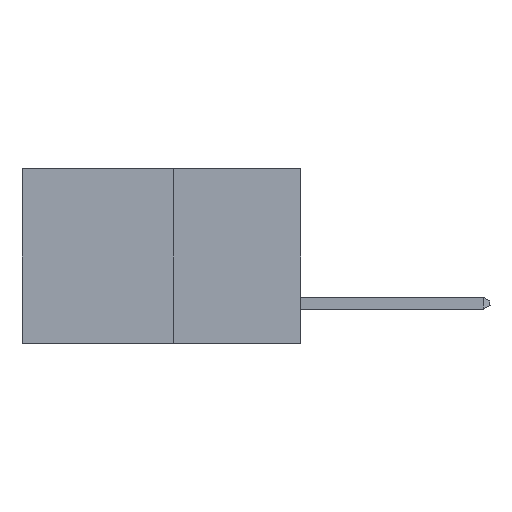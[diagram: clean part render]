
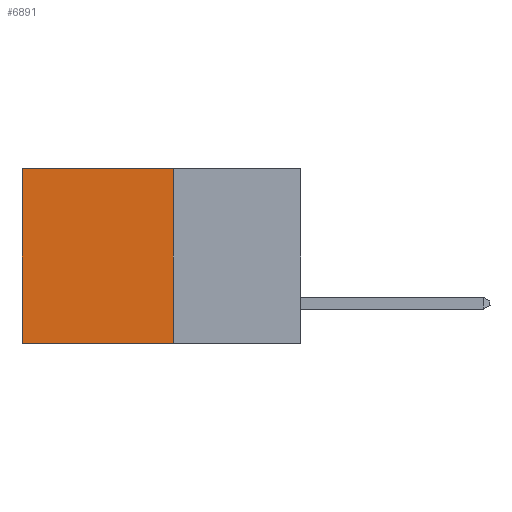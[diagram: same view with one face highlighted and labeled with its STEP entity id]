
A CAD part, left-side view. The second image highlights one B-rep face of the part: STEP entity #6891.
In plain terms, the highlighted planar face has unit normal (-1, 0, 0).
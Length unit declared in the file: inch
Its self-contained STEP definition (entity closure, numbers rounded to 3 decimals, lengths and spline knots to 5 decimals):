
#2284 = CARTESIAN_POINT ( 'NONE',  ( 0.277, 0.59, -0.37 ) ) ;
#2508 = ORIENTED_EDGE ( 'NONE', *, *, #15942, .T. ) ;
#3326 = VECTOR ( 'NONE', #10440, 39.37008 ) ;
#3743 = DIRECTION ( 'NONE',  ( 0., 0., -1. ) ) ;
#4179 = CARTESIAN_POINT ( 'NONE',  ( 0.277, 0.59, 0. ) ) ;
#4608 = FACE_OUTER_BOUND ( 'NONE', #17397, .T. ) ;
#4986 = VECTOR ( 'NONE', #6663, 39.37008 ) ;
#5102 = VERTEX_POINT ( 'NONE', #4179 ) ;
#5275 = CARTESIAN_POINT ( 'NONE',  ( 0.277, 0.27, 0. ) ) ;
#5634 = EDGE_CURVE ( 'NONE', #15242, #12633, #6999, .T. ) ;
#6340 = VECTOR ( 'NONE', #3743, 39.37008 ) ;
#6663 = DIRECTION ( 'NONE',  ( 0., 1., 0. ) ) ;
#6891 = ADVANCED_FACE ( 'NONE', ( #4608 ), #11774, .F. ) ;
#6999 = LINE ( 'NONE', #14785, #3326 ) ;
#7705 = EDGE_CURVE ( 'NONE', #15242, #5102, #15809, .T. ) ;
#9781 = DIRECTION ( 'NONE',  ( 0., 0., -1. ) ) ;
#9804 = DIRECTION ( 'NONE',  ( 1., 0., 0. ) ) ;
#9854 = CARTESIAN_POINT ( 'NONE',  ( 0.277, 0.27, -0.37 ) ) ;
#9985 = LINE ( 'NONE', #15391, #12744 ) ;
#10440 = DIRECTION ( 'NONE',  ( 0., 0., -1. ) ) ;
#10930 = EDGE_CURVE ( 'NONE', #12633, #11135, #9985, .T. ) ;
#11135 = VERTEX_POINT ( 'NONE', #14461 ) ;
#11774 = PLANE ( 'NONE',  #15640 ) ;
#12633 = VERTEX_POINT ( 'NONE', #17826 ) ;
#12744 = VECTOR ( 'NONE', #16720, 39.37008 ) ;
#13635 = LINE ( 'NONE', #2284, #6340 ) ;
#13763 = ORIENTED_EDGE ( 'NONE', *, *, #5634, .F. ) ;
#14461 = CARTESIAN_POINT ( 'NONE',  ( 0.277, 0.59, -0.37 ) ) ;
#14785 = CARTESIAN_POINT ( 'NONE',  ( 0.277, 0.27, -0.37 ) ) ;
#15242 = VERTEX_POINT ( 'NONE', #15780 ) ;
#15391 = CARTESIAN_POINT ( 'NONE',  ( 0.277, 0.27, -0.37 ) ) ;
#15640 = AXIS2_PLACEMENT_3D ( 'NONE', #9854, #9804, #9781 ) ;
#15780 = CARTESIAN_POINT ( 'NONE',  ( 0.277, 0.27, 0. ) ) ;
#15809 = LINE ( 'NONE', #5275, #4986 ) ;
#15942 = EDGE_CURVE ( 'NONE', #5102, #11135, #13635, .T. ) ;
#16720 = DIRECTION ( 'NONE',  ( 0., 1., 0. ) ) ;
#17397 = EDGE_LOOP ( 'NONE', ( #2508, #17867, #13763, #17486 ) ) ;
#17486 = ORIENTED_EDGE ( 'NONE', *, *, #7705, .T. ) ;
#17826 = CARTESIAN_POINT ( 'NONE',  ( 0.277, 0.27, -0.37 ) ) ;
#17867 = ORIENTED_EDGE ( 'NONE', *, *, #10930, .F. ) ;
